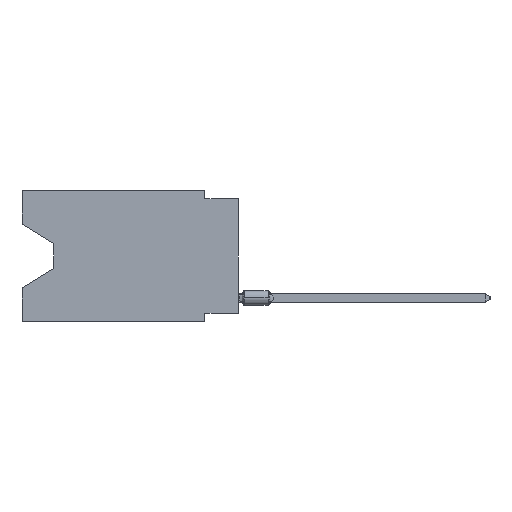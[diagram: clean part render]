
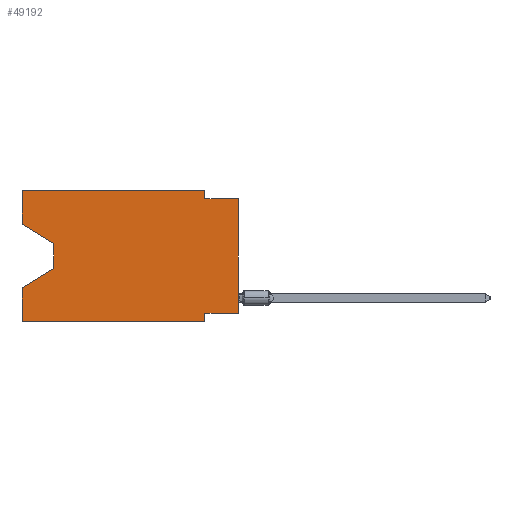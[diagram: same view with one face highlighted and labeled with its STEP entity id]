
A CAD part, left-side view. The second image highlights one B-rep face of the part: STEP entity #49192.
In plain terms, the highlighted planar face has unit normal (-1, 0, 0).
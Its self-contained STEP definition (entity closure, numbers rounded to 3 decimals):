
#762 = DIRECTION ( 'NONE',  ( 0., -0.855, -0.519 ) ) ;
#3113 = DIRECTION ( 'NONE',  ( 0., 0., -1. ) ) ;
#3979 = ORIENTED_EDGE ( 'NONE', *, *, #15380, .F. ) ;
#4645 = VECTOR ( 'NONE', #762, 1000. ) ;
#5455 = CARTESIAN_POINT ( 'NONE',  ( 0., 0., -0.635 ) ) ;
#5983 = VERTEX_POINT ( 'NONE', #27224 ) ;
#6012 = VERTEX_POINT ( 'NONE', #28085 ) ;
#6035 = DIRECTION ( 'NONE',  ( 0., 0., 1. ) ) ;
#6966 = EDGE_CURVE ( 'NONE', #21371, #6012, #41409, .T. ) ;
#7479 = VERTEX_POINT ( 'NONE', #46310 ) ;
#7521 = PLANE ( 'NONE',  #16867 ) ;
#8496 = VECTOR ( 'NONE', #6035, 1000. ) ;
#8999 = EDGE_CURVE ( 'NONE', #7479, #5983, #57912, .T. ) ;
#9175 = CARTESIAN_POINT ( 'NONE',  ( 0., 16.383, 0. ) ) ;
#9341 = CARTESIAN_POINT ( 'NONE',  ( 0., 0., -9.271 ) ) ;
#9504 = VECTOR ( 'NONE', #57616, 1000. ) ;
#10253 = VECTOR ( 'NONE', #17185, 1000. ) ;
#11172 = VECTOR ( 'NONE', #30586, 1000. ) ;
#13075 = EDGE_CURVE ( 'NONE', #34497, #14153, #32659, .T. ) ;
#13115 = VECTOR ( 'NONE', #46372, 1000. ) ;
#14153 = VERTEX_POINT ( 'NONE', #26822 ) ;
#14920 = CARTESIAN_POINT ( 'NONE',  ( 0., 0., -9.271 ) ) ;
#15380 = EDGE_CURVE ( 'NONE', #23090, #47162, #30703, .T. ) ;
#15465 = CARTESIAN_POINT ( 'NONE',  ( 0., 16.383, -2.546 ) ) ;
#16083 = CARTESIAN_POINT ( 'NONE',  ( 0., 0., -0.635 ) ) ;
#16854 = CARTESIAN_POINT ( 'NONE',  ( 0., 13.97, -4.013 ) ) ;
#16867 = AXIS2_PLACEMENT_3D ( 'NONE', #43298, #47117, #3113 ) ;
#16888 = CARTESIAN_POINT ( 'NONE',  ( 0., 13.97, -5.893 ) ) ;
#17185 = DIRECTION ( 'NONE',  ( 0., 0.855, -0.519 ) ) ;
#17876 = EDGE_CURVE ( 'NONE', #48280, #37109, #27752, .T. ) ;
#18649 = ORIENTED_EDGE ( 'NONE', *, *, #17876, .T. ) ;
#20062 = DIRECTION ( 'NONE',  ( 0., 0., -1. ) ) ;
#20485 = VECTOR ( 'NONE', #48304, 1000. ) ;
#21371 = VERTEX_POINT ( 'NONE', #16854 ) ;
#23078 = CARTESIAN_POINT ( 'NONE',  ( 0., 16.383, -2.546 ) ) ;
#23088 = DIRECTION ( 'NONE',  ( 0., -1., 0. ) ) ;
#23090 = VERTEX_POINT ( 'NONE', #37689 ) ;
#23271 = EDGE_CURVE ( 'NONE', #48280, #7479, #45117, .T. ) ;
#23559 = LINE ( 'NONE', #9175, #35342 ) ;
#23889 = ORIENTED_EDGE ( 'NONE', *, *, #37096, .T. ) ;
#24000 = DIRECTION ( 'NONE',  ( 0., 1., 0. ) ) ;
#25159 = LINE ( 'NONE', #5455, #42480 ) ;
#25573 = EDGE_CURVE ( 'NONE', #42955, #31944, #23559, .T. ) ;
#26258 = CARTESIAN_POINT ( 'NONE',  ( 0., 2.54, -9.906 ) ) ;
#26489 = CARTESIAN_POINT ( 'NONE',  ( 0., 16.383, 0. ) ) ;
#26600 = ORIENTED_EDGE ( 'NONE', *, *, #30218, .T. ) ;
#26822 = CARTESIAN_POINT ( 'NONE',  ( 0., 2.54, -0.635 ) ) ;
#27224 = CARTESIAN_POINT ( 'NONE',  ( 0., 2.54, -9.906 ) ) ;
#27514 = VECTOR ( 'NONE', #24000, 1000. ) ;
#27752 = LINE ( 'NONE', #45635, #8496 ) ;
#28053 = LINE ( 'NONE', #16888, #10253 ) ;
#28085 = CARTESIAN_POINT ( 'NONE',  ( 0., 13.97, -5.893 ) ) ;
#29238 = FACE_OUTER_BOUND ( 'NONE', #30597, .T. ) ;
#30218 = EDGE_CURVE ( 'NONE', #42955, #21371, #45346, .T. ) ;
#30420 = CARTESIAN_POINT ( 'NONE',  ( 0., 16.383, 0. ) ) ;
#30586 = DIRECTION ( 'NONE',  ( 0., -1., 0. ) ) ;
#30597 = EDGE_LOOP ( 'NONE', ( #26600, #31768, #56812, #3979, #23889, #48317, #49363, #18649, #38772, #57365, #51818, #52592 ) ) ;
#30703 = LINE ( 'NONE', #30420, #20485 ) ;
#31768 = ORIENTED_EDGE ( 'NONE', *, *, #6966, .T. ) ;
#31944 = VERTEX_POINT ( 'NONE', #46510 ) ;
#32659 = LINE ( 'NONE', #50560, #38088 ) ;
#34236 = LINE ( 'NONE', #46845, #37038 ) ;
#34497 = VERTEX_POINT ( 'NONE', #51040 ) ;
#35101 = EDGE_CURVE ( 'NONE', #14153, #37109, #25159, .T. ) ;
#35342 = VECTOR ( 'NONE', #45529, 1000. ) ;
#36423 = CARTESIAN_POINT ( 'NONE',  ( 0., 13.97, -4.013 ) ) ;
#37038 = VECTOR ( 'NONE', #43322, 1000. ) ;
#37096 = EDGE_CURVE ( 'NONE', #23090, #5983, #34236, .T. ) ;
#37109 = VERTEX_POINT ( 'NONE', #16083 ) ;
#37689 = CARTESIAN_POINT ( 'NONE',  ( 0., 16.383, -9.906 ) ) ;
#38088 = VECTOR ( 'NONE', #20062, 1000. ) ;
#38772 = ORIENTED_EDGE ( 'NONE', *, *, #35101, .F. ) ;
#41409 = LINE ( 'NONE', #36423, #13115 ) ;
#42480 = VECTOR ( 'NONE', #23088, 1000. ) ;
#42955 = VERTEX_POINT ( 'NONE', #15465 ) ;
#43298 = CARTESIAN_POINT ( 'NONE',  ( 0., 16.383, 0. ) ) ;
#43322 = DIRECTION ( 'NONE',  ( 0., -1., 0. ) ) ;
#43390 = CARTESIAN_POINT ( 'NONE',  ( 0., 16.383, -7.36 ) ) ;
#44377 = LINE ( 'NONE', #26489, #11172 ) ;
#45117 = LINE ( 'NONE', #14920, #27514 ) ;
#45346 = LINE ( 'NONE', #23078, #4645 ) ;
#45529 = DIRECTION ( 'NONE',  ( 0., 0., 1. ) ) ;
#45635 = CARTESIAN_POINT ( 'NONE',  ( 0., 0., 0. ) ) ;
#46310 = CARTESIAN_POINT ( 'NONE',  ( 0., 2.54, -9.271 ) ) ;
#46372 = DIRECTION ( 'NONE',  ( 0., 0., -1. ) ) ;
#46510 = CARTESIAN_POINT ( 'NONE',  ( 0., 16.383, 0. ) ) ;
#46845 = CARTESIAN_POINT ( 'NONE',  ( 0., 16.383, -9.906 ) ) ;
#47117 = DIRECTION ( 'NONE',  ( 1., 0., 0. ) ) ;
#47162 = VERTEX_POINT ( 'NONE', #43390 ) ;
#48280 = VERTEX_POINT ( 'NONE', #9341 ) ;
#48304 = DIRECTION ( 'NONE',  ( 0., 0., 1. ) ) ;
#48317 = ORIENTED_EDGE ( 'NONE', *, *, #8999, .F. ) ;
#48479 = EDGE_CURVE ( 'NONE', #31944, #34497, #44377, .T. ) ;
#49192 = ADVANCED_FACE ( 'NONE', ( #29238 ), #7521, .F. ) ;
#49363 = ORIENTED_EDGE ( 'NONE', *, *, #23271, .F. ) ;
#50560 = CARTESIAN_POINT ( 'NONE',  ( 0., 2.54, 0. ) ) ;
#51040 = CARTESIAN_POINT ( 'NONE',  ( 0., 2.54, 0. ) ) ;
#51818 = ORIENTED_EDGE ( 'NONE', *, *, #48479, .F. ) ;
#52592 = ORIENTED_EDGE ( 'NONE', *, *, #25573, .F. ) ;
#54342 = EDGE_CURVE ( 'NONE', #6012, #47162, #28053, .T. ) ;
#56812 = ORIENTED_EDGE ( 'NONE', *, *, #54342, .T. ) ;
#57365 = ORIENTED_EDGE ( 'NONE', *, *, #13075, .F. ) ;
#57616 = DIRECTION ( 'NONE',  ( 0., 0., -1. ) ) ;
#57912 = LINE ( 'NONE', #26258, #9504 ) ;
